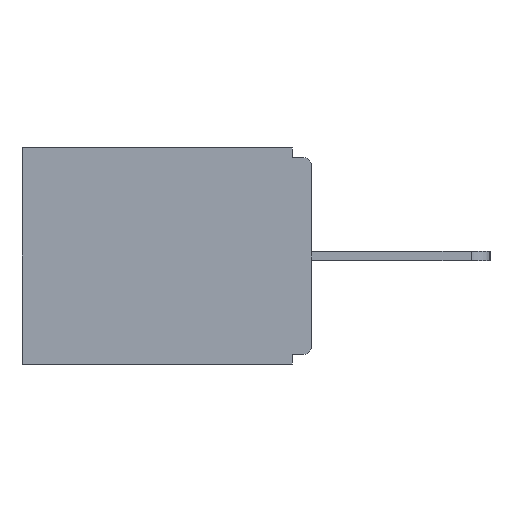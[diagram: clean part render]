
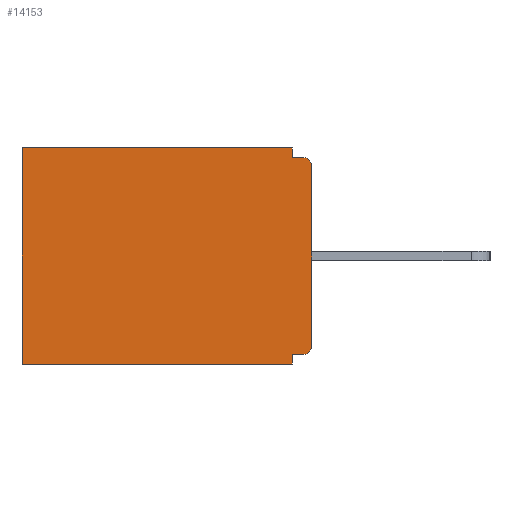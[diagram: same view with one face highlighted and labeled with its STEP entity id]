
A CAD part, left-side view. The second image highlights one B-rep face of the part: STEP entity #14153.
In plain terms, the highlighted planar face has unit normal (-1, 0, 0).
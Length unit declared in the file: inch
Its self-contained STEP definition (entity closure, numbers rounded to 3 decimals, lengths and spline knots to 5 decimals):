
#299 = VERTEX_POINT ( 'NONE', #2348 ) ;
#420 = AXIS2_PLACEMENT_3D ( 'NONE', #729, #1591, #5063 ) ;
#481 = EDGE_CURVE ( 'NONE', #6395, #7054, #9086, .T. ) ;
#570 = VECTOR ( 'NONE', #9799, 39.37008 ) ;
#729 = CARTESIAN_POINT ( 'NONE',  ( 0.298, 0.015, -0.03 ) ) ;
#755 = CARTESIAN_POINT ( 'NONE',  ( 0.298, 0., 0. ) ) ;
#824 = VECTOR ( 'NONE', #4005, 39.37008 ) ;
#1177 = EDGE_CURVE ( 'NONE', #11592, #2449, #5811, .T. ) ;
#1227 = AXIS2_PLACEMENT_3D ( 'NONE', #755, #4239, #14009 ) ;
#1473 = ORIENTED_EDGE ( 'NONE', *, *, #4325, .T. ) ;
#1528 = ORIENTED_EDGE ( 'NONE', *, *, #7504, .F. ) ;
#1591 = DIRECTION ( 'NONE',  ( -1., 0., 0. ) ) ;
#1679 = ORIENTED_EDGE ( 'NONE', *, *, #4215, .T. ) ;
#1756 = PLANE ( 'NONE',  #1227 ) ;
#1817 = FACE_OUTER_BOUND ( 'NONE', #10067, .T. ) ;
#2348 = CARTESIAN_POINT ( 'NONE',  ( 0.298, 0.031, 0. ) ) ;
#2449 = VERTEX_POINT ( 'NONE', #12099 ) ;
#2516 = VERTEX_POINT ( 'NONE', #7924 ) ;
#3019 = EDGE_CURVE ( 'NONE', #11863, #12825, #6467, .T. ) ;
#3070 = CARTESIAN_POINT ( 'NONE',  ( 0.298, 0., 0. ) ) ;
#3185 = DIRECTION ( 'NONE',  ( 0., 0., -1. ) ) ;
#3251 = LINE ( 'NONE', #6476, #12702 ) ;
#3267 = CARTESIAN_POINT ( 'NONE',  ( 0.298, 0.015, -0.015 ) ) ;
#3858 = CARTESIAN_POINT ( 'NONE',  ( 0.298, 0.031, -0.343 ) ) ;
#3891 = ORIENTED_EDGE ( 'NONE', *, *, #7439, .T. ) ;
#4005 = DIRECTION ( 'NONE',  ( 0., 0., -1. ) ) ;
#4215 = EDGE_CURVE ( 'NONE', #11863, #11691, #13807, .T. ) ;
#4239 = DIRECTION ( 'NONE',  ( 1., 0., 0. ) ) ;
#4325 = EDGE_CURVE ( 'NONE', #9607, #2449, #5263, .T. ) ;
#5063 = DIRECTION ( 'NONE',  ( 0., 0., -1. ) ) ;
#5068 = LINE ( 'NONE', #8180, #824 ) ;
#5260 = CARTESIAN_POINT ( 'NONE',  ( 0.298, 0., -0.328 ) ) ;
#5263 = LINE ( 'NONE', #13017, #6914 ) ;
#5466 = ORIENTED_EDGE ( 'NONE', *, *, #8679, .F. ) ;
#5473 = DIRECTION ( 'NONE',  ( 0., 1., 0. ) ) ;
#5580 = VECTOR ( 'NONE', #5473, 39.37008 ) ;
#5767 = ORIENTED_EDGE ( 'NONE', *, *, #1177, .F. ) ;
#5811 = LINE ( 'NONE', #10316, #5580 ) ;
#6063 = DIRECTION ( 'NONE',  ( -1., 0., 0. ) ) ;
#6266 = DIRECTION ( 'NONE',  ( 0., 1., 0. ) ) ;
#6299 = VECTOR ( 'NONE', #6351, 39.37008 ) ;
#6351 = DIRECTION ( 'NONE',  ( 0., 0., -1. ) ) ;
#6395 = VERTEX_POINT ( 'NONE', #12846 ) ;
#6467 = LINE ( 'NONE', #5260, #6877 ) ;
#6476 = CARTESIAN_POINT ( 'NONE',  ( 0.298, 0., 0. ) ) ;
#6643 = ORIENTED_EDGE ( 'NONE', *, *, #6990, .F. ) ;
#6877 = VECTOR ( 'NONE', #6266, 39.37008 ) ;
#6914 = VECTOR ( 'NONE', #3185, 39.37008 ) ;
#6990 = EDGE_CURVE ( 'NONE', #6395, #11691, #11836, .T. ) ;
#7054 = VERTEX_POINT ( 'NONE', #3267 ) ;
#7439 = EDGE_CURVE ( 'NONE', #299, #9607, #3251, .T. ) ;
#7504 = EDGE_CURVE ( 'NONE', #2516, #7054, #11817, .T. ) ;
#7924 = CARTESIAN_POINT ( 'NONE',  ( 0.298, 0.031, -0.015 ) ) ;
#8123 = EDGE_CURVE ( 'NONE', #12825, #11592, #5068, .T. ) ;
#8164 = ORIENTED_EDGE ( 'NONE', *, *, #8123, .F. ) ;
#8180 = CARTESIAN_POINT ( 'NONE',  ( 0.298, 0.031, -0.343 ) ) ;
#8218 = DIRECTION ( 'NONE',  ( 0., 0., -1. ) ) ;
#8572 = CARTESIAN_POINT ( 'NONE',  ( 0.298, 0., -0.015 ) ) ;
#8679 = EDGE_CURVE ( 'NONE', #299, #2516, #10939, .T. ) ;
#8921 = CARTESIAN_POINT ( 'NONE',  ( 0.298, 0.015, -0.328 ) ) ;
#9086 = CIRCLE ( 'NONE', #420, 0.015 ) ;
#9492 = CARTESIAN_POINT ( 'NONE',  ( 0.298, 0.015, -0.313 ) ) ;
#9572 = DIRECTION ( 'NONE',  ( 0., 1., 0. ) ) ;
#9607 = VERTEX_POINT ( 'NONE', #11779 ) ;
#9799 = DIRECTION ( 'NONE',  ( 0., 0., -1. ) ) ;
#9923 = VECTOR ( 'NONE', #12960, 39.37008 ) ;
#10067 = EDGE_LOOP ( 'NONE', ( #11282, #1528, #5466, #3891, #1473, #5767, #8164, #11278, #1679, #6643 ) ) ;
#10316 = CARTESIAN_POINT ( 'NONE',  ( 0.298, 0., -0.343 ) ) ;
#10723 = CARTESIAN_POINT ( 'NONE',  ( 0.298, 0.031, -0.343 ) ) ;
#10919 = CARTESIAN_POINT ( 'NONE',  ( 0.298, 0.031, -0.328 ) ) ;
#10939 = LINE ( 'NONE', #10723, #6299 ) ;
#11278 = ORIENTED_EDGE ( 'NONE', *, *, #3019, .F. ) ;
#11282 = ORIENTED_EDGE ( 'NONE', *, *, #481, .T. ) ;
#11592 = VERTEX_POINT ( 'NONE', #3858 ) ;
#11691 = VERTEX_POINT ( 'NONE', #14054 ) ;
#11779 = CARTESIAN_POINT ( 'NONE',  ( 0.298, 0.46, 0. ) ) ;
#11817 = LINE ( 'NONE', #8572, #9923 ) ;
#11836 = LINE ( 'NONE', #3070, #570 ) ;
#11863 = VERTEX_POINT ( 'NONE', #8921 ) ;
#12099 = CARTESIAN_POINT ( 'NONE',  ( 0.298, 0.46, -0.343 ) ) ;
#12702 = VECTOR ( 'NONE', #9572, 39.37008 ) ;
#12825 = VERTEX_POINT ( 'NONE', #10919 ) ;
#12846 = CARTESIAN_POINT ( 'NONE',  ( 0.298, 0., -0.03 ) ) ;
#12960 = DIRECTION ( 'NONE',  ( 0., -1., 0. ) ) ;
#13017 = CARTESIAN_POINT ( 'NONE',  ( 0.298, 0.46, 0. ) ) ;
#13564 = AXIS2_PLACEMENT_3D ( 'NONE', #9492, #6063, #8218 ) ;
#13807 = CIRCLE ( 'NONE', #13564, 0.015 ) ;
#14009 = DIRECTION ( 'NONE',  ( 0., 0., -1. ) ) ;
#14054 = CARTESIAN_POINT ( 'NONE',  ( 0.298, 0., -0.313 ) ) ;
#14153 = ADVANCED_FACE ( 'NONE', ( #1817 ), #1756, .F. ) ;
